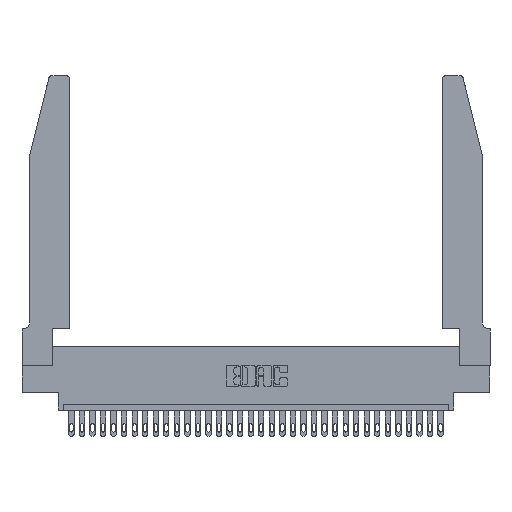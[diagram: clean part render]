
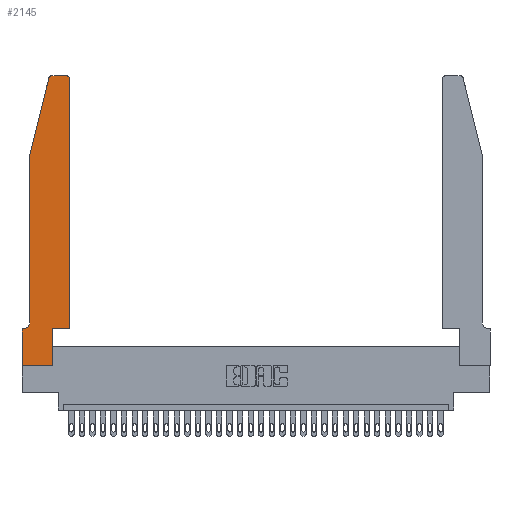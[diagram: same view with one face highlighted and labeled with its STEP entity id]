
A CAD part, top view. The second image highlights one B-rep face of the part: STEP entity #2145.
In plain terms, the highlighted planar face has unit normal (0, 0, 1).
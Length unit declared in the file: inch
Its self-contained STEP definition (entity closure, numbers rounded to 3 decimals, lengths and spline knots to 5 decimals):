
#11 = LINE ( 'NONE', #20908, #28021 ) ;
#495 = DIRECTION ( 'NONE',  ( 1., 0., 0. ) ) ;
#560 = DIRECTION ( 'NONE',  ( 0., 1., 0. ) ) ;
#1511 = ORIENTED_EDGE ( 'NONE', *, *, #23401, .T. ) ;
#1777 = CIRCLE ( 'NONE', #16366, 0.03 ) ;
#2123 = VECTOR ( 'NONE', #14132, 39.37008 ) ;
#2145 = ADVANCED_FACE ( 'NONE', ( #18042 ), #25564, .T. ) ;
#2445 = ORIENTED_EDGE ( 'NONE', *, *, #20456, .T. ) ;
#2768 = EDGE_CURVE ( 'NONE', #9250, #23866, #1777, .T. ) ;
#3040 = ORIENTED_EDGE ( 'NONE', *, *, #31186, .T. ) ;
#3170 = ORIENTED_EDGE ( 'NONE', *, *, #20128, .T. ) ;
#3429 = VECTOR ( 'NONE', #26183, 39.37008 ) ;
#3771 = LINE ( 'NONE', #16454, #30650 ) ;
#4091 = CARTESIAN_POINT ( 'NONE',  ( 0.0755, 2., 0.37 ) ) ;
#4257 = VERTEX_POINT ( 'NONE', #7161 ) ;
#4904 = ORIENTED_EDGE ( 'NONE', *, *, #2768, .T. ) ;
#5288 = LINE ( 'NONE', #4091, #2123 ) ;
#5981 = LINE ( 'NONE', #31029, #28035 ) ;
#6012 = CARTESIAN_POINT ( 'NONE',  ( 0.0755, 0.35, 0.37 ) ) ;
#6840 = VERTEX_POINT ( 'NONE', #32274 ) ;
#7161 = CARTESIAN_POINT ( 'NONE',  ( 0.2865, 0.35, 0.37 ) ) ;
#7268 = ORIENTED_EDGE ( 'NONE', *, *, #10334, .T. ) ;
#7374 = EDGE_CURVE ( 'NONE', #28788, #27502, #3771, .T. ) ;
#7985 = VECTOR ( 'NONE', #560, 39.37008 ) ;
#8090 = CARTESIAN_POINT ( 'NONE',  ( 0.0055, 0.35, 0.37 ) ) ;
#8752 = AXIS2_PLACEMENT_3D ( 'NONE', #15656, #13234, #495 ) ;
#8855 = CARTESIAN_POINT ( 'NONE',  ( 0.284, 2.72, 0.37 ) ) ;
#8978 = DIRECTION ( 'NONE',  ( 0., -1., 0. ) ) ;
#9182 = EDGE_CURVE ( 'NONE', #16538, #4257, #13548, .T. ) ;
#9200 = ORIENTED_EDGE ( 'NONE', *, *, #29383, .T. ) ;
#9250 = VERTEX_POINT ( 'NONE', #10587 ) ;
#10334 = EDGE_CURVE ( 'NONE', #10570, #9250, #32431, .T. ) ;
#10407 = CARTESIAN_POINT ( 'NONE',  ( 0.4505, 0.35, 0.37 ) ) ;
#10464 = LINE ( 'NONE', #28490, #17938 ) ;
#10570 = VERTEX_POINT ( 'NONE', #10407 ) ;
#10587 = CARTESIAN_POINT ( 'NONE',  ( 0.4505, 2.72, 0.37 ) ) ;
#10852 = CARTESIAN_POINT ( 'NONE',  ( 0., 0., 0.37 ) ) ;
#11396 = LINE ( 'NONE', #10852, #14144 ) ;
#11445 = CARTESIAN_POINT ( 'NONE',  ( 0.0055, 0.42, 0.37 ) ) ;
#11451 = VERTEX_POINT ( 'NONE', #22566 ) ;
#11550 = DIRECTION ( 'NONE',  ( -1., 0., 0. ) ) ;
#12039 = DIRECTION ( 'NONE',  ( 0., 0., 1. ) ) ;
#13179 = EDGE_CURVE ( 'NONE', #27502, #14741, #26627, .T. ) ;
#13234 = DIRECTION ( 'NONE',  ( 0., 0., 1. ) ) ;
#13548 = LINE ( 'NONE', #14298, #24982 ) ;
#13605 = CARTESIAN_POINT ( 'NONE',  ( 0.0755, 2., 0.37 ) ) ;
#14132 = DIRECTION ( 'NONE',  ( -0.239, -0.971, 0. ) ) ;
#14144 = VECTOR ( 'NONE', #28678, 39.37008 ) ;
#14298 = CARTESIAN_POINT ( 'NONE',  ( 0.2865, 0.35, 0.37 ) ) ;
#14550 = CARTESIAN_POINT ( 'NONE',  ( 0.4205, 2.72, 0.37 ) ) ;
#14741 = VERTEX_POINT ( 'NONE', #8090 ) ;
#15270 = CARTESIAN_POINT ( 'NONE',  ( 0.25487, 2.72718, 0.37 ) ) ;
#15656 = CARTESIAN_POINT ( 'NONE',  ( 0., 0.35, 0.37 ) ) ;
#15991 = CARTESIAN_POINT ( 'NONE',  ( 0.0755, 0.42, 0.37 ) ) ;
#16205 = DIRECTION ( 'NONE',  ( 1., 0., 0. ) ) ;
#16366 = AXIS2_PLACEMENT_3D ( 'NONE', #14550, #12039, #29682 ) ;
#16454 = CARTESIAN_POINT ( 'NONE',  ( 0.0755, 2., 0.37 ) ) ;
#16538 = VERTEX_POINT ( 'NONE', #24425 ) ;
#16550 = DIRECTION ( 'NONE',  ( 0., -1., 0. ) ) ;
#17229 = ORIENTED_EDGE ( 'NONE', *, *, #19045, .T. ) ;
#17575 = CARTESIAN_POINT ( 'NONE',  ( 0.284, 2.75, 0.37 ) ) ;
#17938 = VECTOR ( 'NONE', #21061, 39.37008 ) ;
#18042 = FACE_OUTER_BOUND ( 'NONE', #30704, .T. ) ;
#18090 = DIRECTION ( 'NONE',  ( 1., 0., 0. ) ) ;
#19045 = EDGE_CURVE ( 'NONE', #6840, #11451, #5981, .T. ) ;
#19257 = LINE ( 'NONE', #6012, #3429 ) ;
#19821 = VERTEX_POINT ( 'NONE', #17575 ) ;
#19878 = AXIS2_PLACEMENT_3D ( 'NONE', #11445, #21528, #11550 ) ;
#20128 = EDGE_CURVE ( 'NONE', #11451, #16538, #11396, .T. ) ;
#20456 = EDGE_CURVE ( 'NONE', #14741, #6840, #19257, .T. ) ;
#20561 = AXIS2_PLACEMENT_3D ( 'NONE', #8855, #26456, #16205 ) ;
#20843 = CARTESIAN_POINT ( 'NONE',  ( 0.4505, 0.35, 0.37 ) ) ;
#20908 = CARTESIAN_POINT ( 'NONE',  ( 0.4505, 0.35, 0.37 ) ) ;
#21061 = DIRECTION ( 'NONE',  ( -1., 0., 0. ) ) ;
#21528 = DIRECTION ( 'NONE',  ( 0., 0., -1. ) ) ;
#22566 = CARTESIAN_POINT ( 'NONE',  ( 0., 0., 0.37 ) ) ;
#23401 = EDGE_CURVE ( 'NONE', #23866, #19821, #10464, .T. ) ;
#23866 = VERTEX_POINT ( 'NONE', #32471 ) ;
#23871 = ORIENTED_EDGE ( 'NONE', *, *, #28801, .T. ) ;
#24425 = CARTESIAN_POINT ( 'NONE',  ( 0.2865, 0., 0.37 ) ) ;
#24982 = VECTOR ( 'NONE', #26774, 39.37008 ) ;
#25564 = PLANE ( 'NONE',  #8752 ) ;
#26183 = DIRECTION ( 'NONE',  ( -1., 0., 0. ) ) ;
#26456 = DIRECTION ( 'NONE',  ( 0., 0., 1. ) ) ;
#26627 = CIRCLE ( 'NONE', #19878, 0.07 ) ;
#26774 = DIRECTION ( 'NONE',  ( 0., 1., 0. ) ) ;
#27407 = ORIENTED_EDGE ( 'NONE', *, *, #9182, .T. ) ;
#27502 = VERTEX_POINT ( 'NONE', #15991 ) ;
#28021 = VECTOR ( 'NONE', #18090, 39.37008 ) ;
#28035 = VECTOR ( 'NONE', #8978, 39.37008 ) ;
#28459 = VERTEX_POINT ( 'NONE', #15270 ) ;
#28490 = CARTESIAN_POINT ( 'NONE',  ( 0.2605, 2.75, 0.37 ) ) ;
#28678 = DIRECTION ( 'NONE',  ( 1., 0., 0. ) ) ;
#28788 = VERTEX_POINT ( 'NONE', #13605 ) ;
#28801 = EDGE_CURVE ( 'NONE', #28459, #28788, #5288, .T. ) ;
#29383 = EDGE_CURVE ( 'NONE', #19821, #28459, #30110, .T. ) ;
#29682 = DIRECTION ( 'NONE',  ( 1., 0., 0. ) ) ;
#30110 = CIRCLE ( 'NONE', #20561, 0.03 ) ;
#30550 = ORIENTED_EDGE ( 'NONE', *, *, #13179, .T. ) ;
#30650 = VECTOR ( 'NONE', #16550, 39.37008 ) ;
#30704 = EDGE_LOOP ( 'NONE', ( #1511, #9200, #23871, #31078, #30550, #2445, #17229, #3170, #27407, #3040, #7268, #4904 ) ) ;
#31029 = CARTESIAN_POINT ( 'NONE',  ( 0., 0., 0.37 ) ) ;
#31078 = ORIENTED_EDGE ( 'NONE', *, *, #7374, .T. ) ;
#31186 = EDGE_CURVE ( 'NONE', #4257, #10570, #11, .T. ) ;
#32274 = CARTESIAN_POINT ( 'NONE',  ( 0., 0.35, 0.37 ) ) ;
#32431 = LINE ( 'NONE', #20843, #7985 ) ;
#32471 = CARTESIAN_POINT ( 'NONE',  ( 0.4205, 2.75, 0.37 ) ) ;
